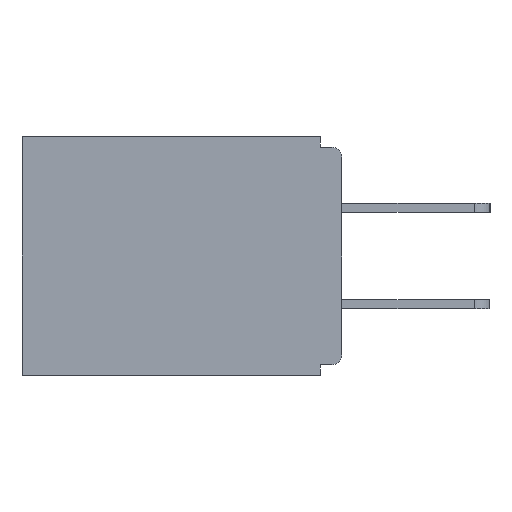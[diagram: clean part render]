
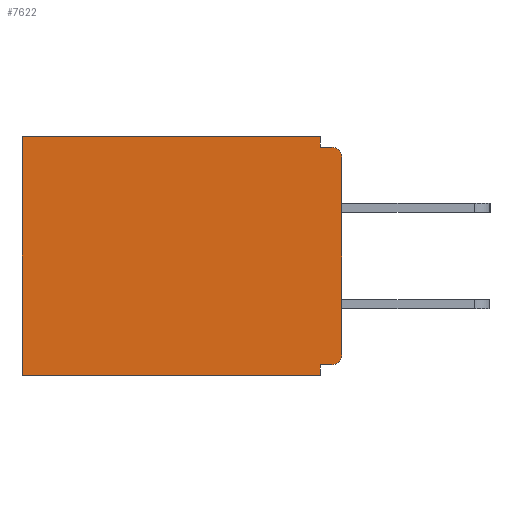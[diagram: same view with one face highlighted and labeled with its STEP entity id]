
A CAD part, left-side view. The second image highlights one B-rep face of the part: STEP entity #7622.
In plain terms, the highlighted planar face has unit normal (-1, 0, 0).
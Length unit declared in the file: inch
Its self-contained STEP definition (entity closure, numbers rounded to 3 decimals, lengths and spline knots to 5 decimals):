
#30 = CARTESIAN_POINT ( 'NONE',  ( 0.298, 0.031, -0.015 ) ) ;
#46 = VECTOR ( 'NONE', #6494, 39.37008 ) ;
#186 = CARTESIAN_POINT ( 'NONE',  ( 0.298, 0.46, 0. ) ) ;
#264 = VERTEX_POINT ( 'NONE', #10637 ) ;
#526 = CARTESIAN_POINT ( 'NONE',  ( 0.298, 0.031, -0.343 ) ) ;
#747 = DIRECTION ( 'NONE',  ( 0., 1., 0. ) ) ;
#967 = ORIENTED_EDGE ( 'NONE', *, *, #8225, .F. ) ;
#1833 = CIRCLE ( 'NONE', #2896, 0.015 ) ;
#1899 = LINE ( 'NONE', #5337, #10998 ) ;
#1964 = ORIENTED_EDGE ( 'NONE', *, *, #8761, .T. ) ;
#1981 = VECTOR ( 'NONE', #11773, 39.37008 ) ;
#2398 = VECTOR ( 'NONE', #7288, 39.37008 ) ;
#2631 = CARTESIAN_POINT ( 'NONE',  ( 0.298, 0., 0. ) ) ;
#2888 = CARTESIAN_POINT ( 'NONE',  ( 0.298, 0., -0.328 ) ) ;
#2896 = AXIS2_PLACEMENT_3D ( 'NONE', #14948, #7962, #11256 ) ;
#3259 = ORIENTED_EDGE ( 'NONE', *, *, #14356, .T. ) ;
#3391 = VECTOR ( 'NONE', #3597, 39.37008 ) ;
#3429 = CARTESIAN_POINT ( 'NONE',  ( 0.298, 0.015, -0.03 ) ) ;
#3597 = DIRECTION ( 'NONE',  ( 0., -1., 0. ) ) ;
#3887 = LINE ( 'NONE', #2888, #46 ) ;
#4357 = EDGE_CURVE ( 'NONE', #14326, #8449, #7561, .T. ) ;
#4764 = PLANE ( 'NONE',  #15191 ) ;
#4783 = LINE ( 'NONE', #2631, #15136 ) ;
#4832 = VERTEX_POINT ( 'NONE', #7673 ) ;
#4918 = ORIENTED_EDGE ( 'NONE', *, *, #13379, .T. ) ;
#4973 = EDGE_LOOP ( 'NONE', ( #9460, #9283, #13917, #3259, #4918, #8493, #14842, #967, #1964, #15242 ) ) ;
#5337 = CARTESIAN_POINT ( 'NONE',  ( 0.298, 0., -0.343 ) ) ;
#5497 = DIRECTION ( 'NONE',  ( -1., 0., 0. ) ) ;
#5739 = CARTESIAN_POINT ( 'NONE',  ( 0.298, 0., -0.313 ) ) ;
#6199 = CARTESIAN_POINT ( 'NONE',  ( 0.298, 0.031, -0.343 ) ) ;
#6442 = VERTEX_POINT ( 'NONE', #11474 ) ;
#6494 = DIRECTION ( 'NONE',  ( 0., 1., 0. ) ) ;
#6551 = VERTEX_POINT ( 'NONE', #5739 ) ;
#7106 = VERTEX_POINT ( 'NONE', #526 ) ;
#7236 = CARTESIAN_POINT ( 'NONE',  ( 0.298, 0., 0. ) ) ;
#7288 = DIRECTION ( 'NONE',  ( 0., 0., -1. ) ) ;
#7561 = LINE ( 'NONE', #9555, #1981 ) ;
#7622 = ADVANCED_FACE ( 'NONE', ( #12987 ), #4764, .F. ) ;
#7625 = VERTEX_POINT ( 'NONE', #186 ) ;
#7673 = CARTESIAN_POINT ( 'NONE',  ( 0.298, 0.46, -0.343 ) ) ;
#7962 = DIRECTION ( 'NONE',  ( -1., 0., 0. ) ) ;
#8109 = DIRECTION ( 'NONE',  ( 0., 0., -1. ) ) ;
#8225 = EDGE_CURVE ( 'NONE', #8830, #12119, #3887, .T. ) ;
#8447 = CARTESIAN_POINT ( 'NONE',  ( 0.298, 0.46, 0. ) ) ;
#8449 = VERTEX_POINT ( 'NONE', #30 ) ;
#8493 = ORIENTED_EDGE ( 'NONE', *, *, #11220, .F. ) ;
#8527 = EDGE_CURVE ( 'NONE', #12119, #7106, #10029, .T. ) ;
#8761 = EDGE_CURVE ( 'NONE', #8830, #6551, #1833, .T. ) ;
#8830 = VERTEX_POINT ( 'NONE', #11653 ) ;
#9283 = ORIENTED_EDGE ( 'NONE', *, *, #12405, .F. ) ;
#9288 = VECTOR ( 'NONE', #13407, 39.37008 ) ;
#9460 = ORIENTED_EDGE ( 'NONE', *, *, #11802, .T. ) ;
#9555 = CARTESIAN_POINT ( 'NONE',  ( 0.298, 0.031, -0.343 ) ) ;
#9696 = DIRECTION ( 'NONE',  ( 0., 0., -1. ) ) ;
#9697 = LINE ( 'NONE', #14403, #3391 ) ;
#9805 = AXIS2_PLACEMENT_3D ( 'NONE', #3429, #5497, #8109 ) ;
#10029 = LINE ( 'NONE', #6199, #9288 ) ;
#10637 = CARTESIAN_POINT ( 'NONE',  ( 0.298, 0., -0.03 ) ) ;
#10757 = CARTESIAN_POINT ( 'NONE',  ( 0.298, 0., 0. ) ) ;
#10947 = CARTESIAN_POINT ( 'NONE',  ( 0.298, 0.031, 0. ) ) ;
#10998 = VECTOR ( 'NONE', #747, 39.37008 ) ;
#11180 = EDGE_CURVE ( 'NONE', #264, #6551, #14502, .T. ) ;
#11220 = EDGE_CURVE ( 'NONE', #7106, #4832, #1899, .T. ) ;
#11256 = DIRECTION ( 'NONE',  ( 0., 0., -1. ) ) ;
#11474 = CARTESIAN_POINT ( 'NONE',  ( 0.298, 0.015, -0.015 ) ) ;
#11653 = CARTESIAN_POINT ( 'NONE',  ( 0.298, 0.015, -0.328 ) ) ;
#11773 = DIRECTION ( 'NONE',  ( 0., 0., -1. ) ) ;
#11802 = EDGE_CURVE ( 'NONE', #264, #6442, #14318, .T. ) ;
#11963 = DIRECTION ( 'NONE',  ( 1., 0., 0. ) ) ;
#12048 = LINE ( 'NONE', #8447, #2398 ) ;
#12119 = VERTEX_POINT ( 'NONE', #14586 ) ;
#12405 = EDGE_CURVE ( 'NONE', #8449, #6442, #9697, .T. ) ;
#12987 = FACE_OUTER_BOUND ( 'NONE', #4973, .T. ) ;
#13005 = VECTOR ( 'NONE', #13595, 39.37008 ) ;
#13306 = DIRECTION ( 'NONE',  ( 0., 1., 0. ) ) ;
#13379 = EDGE_CURVE ( 'NONE', #7625, #4832, #12048, .T. ) ;
#13407 = DIRECTION ( 'NONE',  ( 0., 0., -1. ) ) ;
#13595 = DIRECTION ( 'NONE',  ( 0., 0., -1. ) ) ;
#13917 = ORIENTED_EDGE ( 'NONE', *, *, #4357, .F. ) ;
#14318 = CIRCLE ( 'NONE', #9805, 0.015 ) ;
#14326 = VERTEX_POINT ( 'NONE', #10947 ) ;
#14356 = EDGE_CURVE ( 'NONE', #14326, #7625, #4783, .T. ) ;
#14403 = CARTESIAN_POINT ( 'NONE',  ( 0.298, 0., -0.015 ) ) ;
#14502 = LINE ( 'NONE', #10757, #13005 ) ;
#14586 = CARTESIAN_POINT ( 'NONE',  ( 0.298, 0.031, -0.328 ) ) ;
#14842 = ORIENTED_EDGE ( 'NONE', *, *, #8527, .F. ) ;
#14948 = CARTESIAN_POINT ( 'NONE',  ( 0.298, 0.015, -0.313 ) ) ;
#15136 = VECTOR ( 'NONE', #13306, 39.37008 ) ;
#15191 = AXIS2_PLACEMENT_3D ( 'NONE', #7236, #11963, #9696 ) ;
#15242 = ORIENTED_EDGE ( 'NONE', *, *, #11180, .F. ) ;
